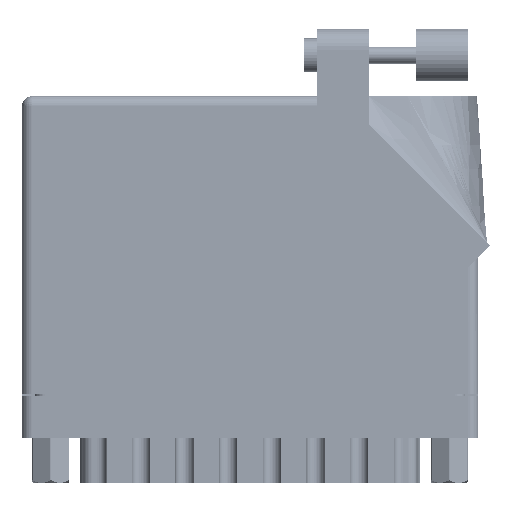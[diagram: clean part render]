
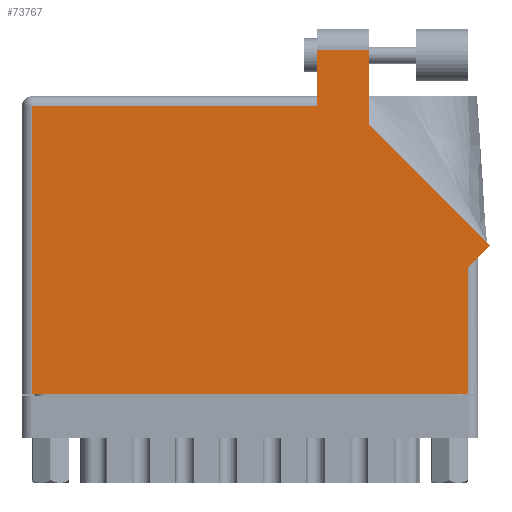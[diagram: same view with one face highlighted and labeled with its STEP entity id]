
A CAD part, front view. The second image highlights one B-rep face of the part: STEP entity #73767.
In plain terms, the highlighted face is planar.
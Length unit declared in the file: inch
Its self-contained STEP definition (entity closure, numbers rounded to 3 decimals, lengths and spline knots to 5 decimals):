
#799 = VECTOR ( 'NONE', #30569, 39.37008 ) ;
#2699 = VERTEX_POINT ( 'NONE', #17494 ) ;
#8661 = DIRECTION ( 'NONE',  ( -0.707, 0.707, 0. ) ) ;
#9521 = LINE ( 'NONE', #22016, #36598 ) ;
#10077 = DIRECTION ( 'NONE',  ( 0., -1., 0. ) ) ;
#10944 = CARTESIAN_POINT ( 'NONE',  ( 1.758, 2.05, 0. ) ) ;
#11623 = EDGE_CURVE ( 'NONE', #51068, #72096, #71069, .T. ) ;
#11665 = ORIENTED_EDGE ( 'NONE', *, *, #64079, .T. ) ;
#12959 = LINE ( 'NONE', #17074, #43177 ) ;
#13670 = EDGE_CURVE ( 'NONE', #33110, #20688, #9521, .T. ) ;
#14388 = VERTEX_POINT ( 'NONE', #82220 ) ;
#14750 = CARTESIAN_POINT ( 'NONE',  ( 2.656, 0.815, 0. ) ) ;
#15183 = CARTESIAN_POINT ( 'NONE',  ( 2.656, 0., 0. ) ) ;
#15880 = DIRECTION ( 'NONE',  ( 0., 1., 0. ) ) ;
#15989 = AXIS2_PLACEMENT_3D ( 'NONE', #23826, #57487, #17652 ) ;
#16081 = EDGE_CURVE ( 'NONE', #14388, #24288, #18425, .T. ) ;
#17074 = CARTESIAN_POINT ( 'NONE',  ( 2.718, 0.815, 0. ) ) ;
#17494 = CARTESIAN_POINT ( 'NONE',  ( 2.78871, 0.88571, 0. ) ) ;
#17652 = DIRECTION ( 'NONE',  ( -1., 0., 0. ) ) ;
#18135 = VERTEX_POINT ( 'NONE', #78939 ) ;
#18425 = LINE ( 'NONE', #43624, #799 ) ;
#19410 = FACE_OUTER_BOUND ( 'NONE', #20917, .T. ) ;
#20072 = VECTOR ( 'NONE', #10077, 39.37008 ) ;
#20562 = CARTESIAN_POINT ( 'NONE',  ( 2.78871, 0.88571, 0. ) ) ;
#20688 = VERTEX_POINT ( 'NONE', #34440 ) ;
#20917 = EDGE_LOOP ( 'NONE', ( #78408, #11665, #81060, #75997, #83641, #31201, #79115, #51924, #45369 ) ) ;
#22016 = CARTESIAN_POINT ( 'NONE',  ( 2.065, 1.60942, 0. ) ) ;
#22884 = CARTESIAN_POINT ( 'NONE',  ( 1.758, 1.775, 0. ) ) ;
#23826 = CARTESIAN_POINT ( 'NONE',  ( 0., 1.775, 0. ) ) ;
#24288 = VERTEX_POINT ( 'NONE', #15183 ) ;
#25051 = LINE ( 'NONE', #44458, #67774 ) ;
#30163 = LINE ( 'NONE', #20562, #45757 ) ;
#30270 = VECTOR ( 'NONE', #51584, 39.37008 ) ;
#30569 = DIRECTION ( 'NONE',  ( 1., 0., 0. ) ) ;
#31201 = ORIENTED_EDGE ( 'NONE', *, *, #16081, .T. ) ;
#32086 = CARTESIAN_POINT ( 'NONE',  ( 2.065, 1.60942, 0. ) ) ;
#32185 = CARTESIAN_POINT ( 'NONE',  ( 2.656, 0.753, 0. ) ) ;
#33110 = VERTEX_POINT ( 'NONE', #32086 ) ;
#34311 = LINE ( 'NONE', #14750, #46797 ) ;
#34440 = CARTESIAN_POINT ( 'NONE',  ( 2.065, 2.05, 0. ) ) ;
#36598 = VECTOR ( 'NONE', #15880, 39.37008 ) ;
#36664 = EDGE_CURVE ( 'NONE', #2699, #33110, #30163, .T. ) ;
#43177 = VECTOR ( 'NONE', #70624, 39.37008 ) ;
#43624 = CARTESIAN_POINT ( 'NONE',  ( 0., 0., 0. ) ) ;
#44458 = CARTESIAN_POINT ( 'NONE',  ( 0.062, 0., 0. ) ) ;
#44931 = CARTESIAN_POINT ( 'NONE',  ( 0., 1.713, 0. ) ) ;
#45369 = ORIENTED_EDGE ( 'NONE', *, *, #36664, .T. ) ;
#45757 = VECTOR ( 'NONE', #8661, 39.37008 ) ;
#46797 = VECTOR ( 'NONE', #74025, 39.37008 ) ;
#47944 = LINE ( 'NONE', #44931, #30270 ) ;
#49431 = EDGE_CURVE ( 'NONE', #76473, #2699, #12959, .T. ) ;
#51052 = DIRECTION ( 'NONE',  ( -1., 0., 0. ) ) ;
#51068 = VERTEX_POINT ( 'NONE', #56519 ) ;
#51584 = DIRECTION ( 'NONE',  ( -1., 0., 0. ) ) ;
#51924 = ORIENTED_EDGE ( 'NONE', *, *, #49431, .T. ) ;
#53771 = EDGE_CURVE ( 'NONE', #24288, #76473, #34311, .T. ) ;
#55388 = CARTESIAN_POINT ( 'NONE',  ( 1.758, 1.713, 0. ) ) ;
#56519 = CARTESIAN_POINT ( 'NONE',  ( 1.758, 2.05, 0. ) ) ;
#57487 = DIRECTION ( 'NONE',  ( 0., 0., -1. ) ) ;
#57747 = DIRECTION ( 'NONE',  ( 0., -1., 0. ) ) ;
#59505 = EDGE_CURVE ( 'NONE', #18135, #14388, #25051, .T. ) ;
#60002 = EDGE_CURVE ( 'NONE', #72096, #18135, #47944, .T. ) ;
#63911 = PLANE ( 'NONE',  #15989 ) ;
#64079 = EDGE_CURVE ( 'NONE', #20688, #51068, #77363, .T. ) ;
#67774 = VECTOR ( 'NONE', #57747, 39.37008 ) ;
#70624 = DIRECTION ( 'NONE',  ( 0.707, 0.707, 0. ) ) ;
#71069 = LINE ( 'NONE', #22884, #20072 ) ;
#72096 = VERTEX_POINT ( 'NONE', #55388 ) ;
#73199 = VECTOR ( 'NONE', #51052, 39.37008 ) ;
#73767 = ADVANCED_FACE ( 'NONE', ( #19410 ), #63911, .F. ) ;
#74025 = DIRECTION ( 'NONE',  ( 0., 1., 0. ) ) ;
#75997 = ORIENTED_EDGE ( 'NONE', *, *, #60002, .T. ) ;
#76473 = VERTEX_POINT ( 'NONE', #32185 ) ;
#77363 = LINE ( 'NONE', #10944, #73199 ) ;
#78408 = ORIENTED_EDGE ( 'NONE', *, *, #13670, .T. ) ;
#78939 = CARTESIAN_POINT ( 'NONE',  ( 0.062, 1.713, 0. ) ) ;
#79115 = ORIENTED_EDGE ( 'NONE', *, *, #53771, .T. ) ;
#81060 = ORIENTED_EDGE ( 'NONE', *, *, #11623, .T. ) ;
#82220 = CARTESIAN_POINT ( 'NONE',  ( 0.062, 0., 0. ) ) ;
#83641 = ORIENTED_EDGE ( 'NONE', *, *, #59505, .T. ) ;
